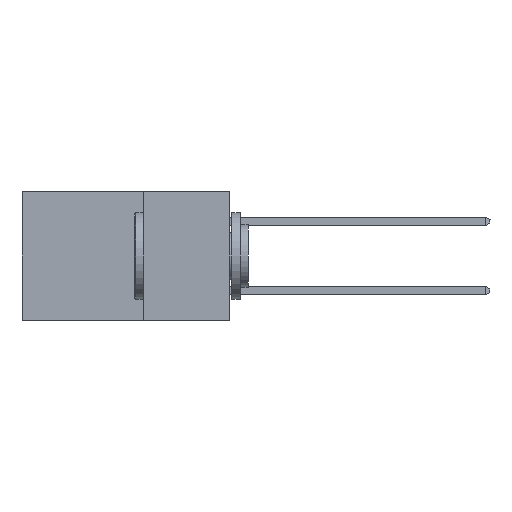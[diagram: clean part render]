
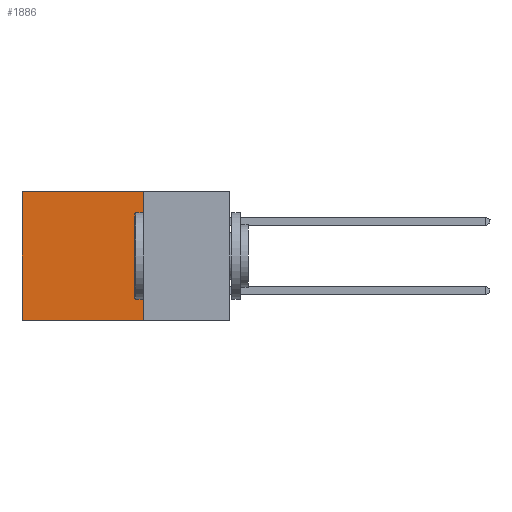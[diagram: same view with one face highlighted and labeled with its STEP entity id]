
A CAD part, left-side view. The second image highlights one B-rep face of the part: STEP entity #1886.
In plain terms, the highlighted planar face has unit normal (-1, 0, 0).
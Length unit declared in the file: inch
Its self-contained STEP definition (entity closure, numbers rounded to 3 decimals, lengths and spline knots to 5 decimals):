
#10 = LINE ( 'NONE', #19185, #7334 ) ;
#436 = ORIENTED_EDGE ( 'NONE', *, *, #5511, .T. ) ;
#656 = VERTEX_POINT ( 'NONE', #12290 ) ;
#745 = CARTESIAN_POINT ( 'NONE',  ( 0.298, 0.6, 0. ) ) ;
#1556 = EDGE_CURVE ( 'NONE', #20838, #656, #5419, .T. ) ;
#1798 = VECTOR ( 'NONE', #21326, 39.37008 ) ;
#1886 = ADVANCED_FACE ( 'NONE', ( #12211 ), #13299, .F. ) ;
#2276 = CARTESIAN_POINT ( 'NONE',  ( 0.298, 0.25, -0.37 ) ) ;
#3154 = CARTESIAN_POINT ( 'NONE',  ( 0.298, 0.25, 0. ) ) ;
#3451 = VECTOR ( 'NONE', #5623, 39.37008 ) ;
#4335 = LINE ( 'NONE', #13345, #4575 ) ;
#4575 = VECTOR ( 'NONE', #15063, 39.37008 ) ;
#5313 = ORIENTED_EDGE ( 'NONE', *, *, #1556, .T. ) ;
#5419 = LINE ( 'NONE', #13177, #1798 ) ;
#5511 = EDGE_CURVE ( 'NONE', #6568, #20838, #4335, .T. ) ;
#5623 = DIRECTION ( 'NONE',  ( 0., 1., 0. ) ) ;
#6049 = LINE ( 'NONE', #2276, #3451 ) ;
#6568 = VERTEX_POINT ( 'NONE', #8333 ) ;
#7334 = VECTOR ( 'NONE', #17804, 39.37008 ) ;
#8036 = EDGE_CURVE ( 'NONE', #14456, #656, #6049, .T. ) ;
#8333 = CARTESIAN_POINT ( 'NONE',  ( 0.298, 0.25, 0. ) ) ;
#8449 = EDGE_CURVE ( 'NONE', #6568, #14456, #10, .T. ) ;
#9863 = DIRECTION ( 'NONE',  ( 1., 0., 0. ) ) ;
#11826 = EDGE_LOOP ( 'NONE', ( #5313, #18733, #19075, #436 ) ) ;
#12211 = FACE_OUTER_BOUND ( 'NONE', #11826, .T. ) ;
#12290 = CARTESIAN_POINT ( 'NONE',  ( 0.298, 0.6, -0.37 ) ) ;
#13177 = CARTESIAN_POINT ( 'NONE',  ( 0.298, 0.6, 0. ) ) ;
#13299 = PLANE ( 'NONE',  #20030 ) ;
#13345 = CARTESIAN_POINT ( 'NONE',  ( 0.298, 0.25, 0. ) ) ;
#14456 = VERTEX_POINT ( 'NONE', #18445 ) ;
#15063 = DIRECTION ( 'NONE',  ( 0., 1., 0. ) ) ;
#16661 = DIRECTION ( 'NONE',  ( 0., 0., -1. ) ) ;
#17804 = DIRECTION ( 'NONE',  ( 0., 0., -1. ) ) ;
#18445 = CARTESIAN_POINT ( 'NONE',  ( 0.298, 0.25, -0.37 ) ) ;
#18733 = ORIENTED_EDGE ( 'NONE', *, *, #8036, .F. ) ;
#19075 = ORIENTED_EDGE ( 'NONE', *, *, #8449, .F. ) ;
#19185 = CARTESIAN_POINT ( 'NONE',  ( 0.298, 0.25, 0. ) ) ;
#20030 = AXIS2_PLACEMENT_3D ( 'NONE', #3154, #9863, #16661 ) ;
#20838 = VERTEX_POINT ( 'NONE', #745 ) ;
#21326 = DIRECTION ( 'NONE',  ( 0., 0., -1. ) ) ;
